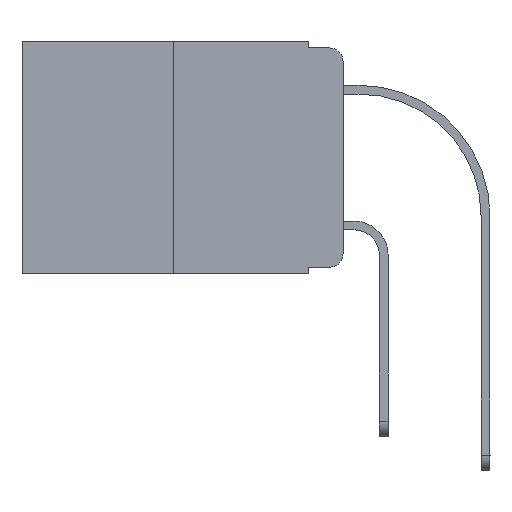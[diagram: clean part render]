
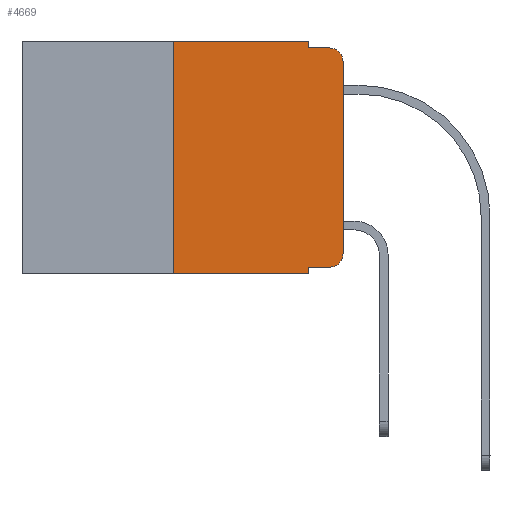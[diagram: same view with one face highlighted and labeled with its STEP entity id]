
A CAD part, left-side view. The second image highlights one B-rep face of the part: STEP entity #4669.
In plain terms, the highlighted planar face has unit normal (-1, 0, 0).
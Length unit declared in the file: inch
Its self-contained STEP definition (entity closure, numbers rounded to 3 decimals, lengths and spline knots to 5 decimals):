
#262 = DIRECTION ( 'NONE',  ( 0., 0., -1. ) ) ;
#368 = CIRCLE ( 'NONE', #6125, 0.02 ) ;
#521 = DIRECTION ( 'NONE',  ( 0., -1., 0. ) ) ;
#764 = CARTESIAN_POINT ( 'NONE',  ( 0., 0.25, 0. ) ) ;
#827 = EDGE_CURVE ( 'NONE', #19332, #5229, #12597, .T. ) ;
#1513 = VERTEX_POINT ( 'NONE', #13084 ) ;
#1625 = EDGE_CURVE ( 'NONE', #12214, #4567, #8659, .T. ) ;
#1886 = CIRCLE ( 'NONE', #13680, 0.02 ) ;
#1904 = VECTOR ( 'NONE', #11044, 39.37008 ) ;
#2000 = CARTESIAN_POINT ( 'NONE',  ( 0., 0.051, -0.333 ) ) ;
#2262 = EDGE_CURVE ( 'NONE', #12214, #17678, #7145, .T. ) ;
#3136 = DIRECTION ( 'NONE',  ( 0., -1., 0. ) ) ;
#3420 = ORIENTED_EDGE ( 'NONE', *, *, #6524, .F. ) ;
#3821 = CARTESIAN_POINT ( 'NONE',  ( 0., 0., -0.03 ) ) ;
#3942 = LINE ( 'NONE', #16697, #20056 ) ;
#4567 = VERTEX_POINT ( 'NONE', #17156 ) ;
#4573 = DIRECTION ( 'NONE',  ( 0., 0., 1. ) ) ;
#4669 = ADVANCED_FACE ( 'NONE', ( #4906 ), #11142, .F. ) ;
#4838 = VERTEX_POINT ( 'NONE', #14924 ) ;
#4906 = FACE_OUTER_BOUND ( 'NONE', #20108, .T. ) ;
#5229 = VERTEX_POINT ( 'NONE', #764 ) ;
#5810 = EDGE_CURVE ( 'NONE', #5229, #1513, #15790, .T. ) ;
#6083 = DIRECTION ( 'NONE',  ( 0., -1., 0. ) ) ;
#6125 = AXIS2_PLACEMENT_3D ( 'NONE', #7836, #12792, #10896 ) ;
#6155 = DIRECTION ( 'NONE',  ( 0., 0., -1. ) ) ;
#6524 = EDGE_CURVE ( 'NONE', #1513, #15358, #3942, .T. ) ;
#6560 = VECTOR ( 'NONE', #14799, 39.37008 ) ;
#7093 = DIRECTION ( 'NONE',  ( 0., 0., -1. ) ) ;
#7145 = LINE ( 'NONE', #9455, #1904 ) ;
#7532 = DIRECTION ( 'NONE',  ( 0., -1., 0. ) ) ;
#7761 = VERTEX_POINT ( 'NONE', #11628 ) ;
#7836 = CARTESIAN_POINT ( 'NONE',  ( 0., 0.02, -0.03 ) ) ;
#8020 = ORIENTED_EDGE ( 'NONE', *, *, #5810, .F. ) ;
#8023 = CARTESIAN_POINT ( 'NONE',  ( 0., 0.25, -0.343 ) ) ;
#8470 = CARTESIAN_POINT ( 'NONE',  ( 0., 0., 0. ) ) ;
#8659 = LINE ( 'NONE', #2000, #18472 ) ;
#9040 = EDGE_CURVE ( 'NONE', #4838, #12448, #11527, .T. ) ;
#9397 = ORIENTED_EDGE ( 'NONE', *, *, #20646, .F. ) ;
#9430 = ORIENTED_EDGE ( 'NONE', *, *, #827, .F. ) ;
#9455 = CARTESIAN_POINT ( 'NONE',  ( 0., 0.051, 0. ) ) ;
#10097 = ORIENTED_EDGE ( 'NONE', *, *, #9040, .T. ) ;
#10896 = DIRECTION ( 'NONE',  ( 0., 0., -1. ) ) ;
#11007 = ORIENTED_EDGE ( 'NONE', *, *, #11699, .T. ) ;
#11044 = DIRECTION ( 'NONE',  ( 0., 0., -1. ) ) ;
#11142 = PLANE ( 'NONE',  #19869 ) ;
#11153 = LINE ( 'NONE', #15801, #12660 ) ;
#11527 = LINE ( 'NONE', #8470, #6560 ) ;
#11628 = CARTESIAN_POINT ( 'NONE',  ( 0., 0.02, -0.01 ) ) ;
#11699 = EDGE_CURVE ( 'NONE', #19332, #17678, #11153, .T. ) ;
#12214 = VERTEX_POINT ( 'NONE', #13014 ) ;
#12390 = CARTESIAN_POINT ( 'NONE',  ( 0., 0.25, 0. ) ) ;
#12448 = VERTEX_POINT ( 'NONE', #3821 ) ;
#12595 = CARTESIAN_POINT ( 'NONE',  ( 0., 0.051, -0.01 ) ) ;
#12597 = LINE ( 'NONE', #12390, #19564 ) ;
#12660 = VECTOR ( 'NONE', #3136, 39.37008 ) ;
#12699 = CARTESIAN_POINT ( 'NONE',  ( 0., 0.051, -0.01 ) ) ;
#12792 = DIRECTION ( 'NONE',  ( -1., 0., 0. ) ) ;
#13014 = CARTESIAN_POINT ( 'NONE',  ( 0., 0.051, -0.333 ) ) ;
#13084 = CARTESIAN_POINT ( 'NONE',  ( 0., 0.051, 0. ) ) ;
#13507 = ORIENTED_EDGE ( 'NONE', *, *, #2262, .F. ) ;
#13570 = DIRECTION ( 'NONE',  ( -1., 0., 0. ) ) ;
#13680 = AXIS2_PLACEMENT_3D ( 'NONE', #15755, #13570, #6155 ) ;
#13827 = ORIENTED_EDGE ( 'NONE', *, *, #18657, .T. ) ;
#14082 = EDGE_CURVE ( 'NONE', #12448, #7761, #368, .T. ) ;
#14799 = DIRECTION ( 'NONE',  ( 0., 0., 1. ) ) ;
#14924 = CARTESIAN_POINT ( 'NONE',  ( 0., 0., -0.313 ) ) ;
#15358 = VERTEX_POINT ( 'NONE', #12699 ) ;
#15474 = CARTESIAN_POINT ( 'NONE',  ( 0., 0.473, 0. ) ) ;
#15719 = ORIENTED_EDGE ( 'NONE', *, *, #1625, .T. ) ;
#15755 = CARTESIAN_POINT ( 'NONE',  ( 0., 0.02, -0.313 ) ) ;
#15790 = LINE ( 'NONE', #15474, #18036 ) ;
#15801 = CARTESIAN_POINT ( 'NONE',  ( 0., 0.473, -0.343 ) ) ;
#16697 = CARTESIAN_POINT ( 'NONE',  ( 0., 0.051, 0. ) ) ;
#17156 = CARTESIAN_POINT ( 'NONE',  ( 0., 0.02, -0.333 ) ) ;
#17483 = ORIENTED_EDGE ( 'NONE', *, *, #14082, .T. ) ;
#17567 = DIRECTION ( 'NONE',  ( 1., 0., 0. ) ) ;
#17678 = VERTEX_POINT ( 'NONE', #19740 ) ;
#17782 = CARTESIAN_POINT ( 'NONE',  ( 0., 0.473, 0. ) ) ;
#17821 = VECTOR ( 'NONE', #7532, 39.37008 ) ;
#18036 = VECTOR ( 'NONE', #6083, 39.37008 ) ;
#18472 = VECTOR ( 'NONE', #521, 39.37008 ) ;
#18657 = EDGE_CURVE ( 'NONE', #4567, #4838, #1886, .T. ) ;
#19332 = VERTEX_POINT ( 'NONE', #8023 ) ;
#19564 = VECTOR ( 'NONE', #4573, 39.37008 ) ;
#19740 = CARTESIAN_POINT ( 'NONE',  ( 0., 0.051, -0.343 ) ) ;
#19869 = AXIS2_PLACEMENT_3D ( 'NONE', #17782, #17567, #262 ) ;
#20056 = VECTOR ( 'NONE', #7093, 39.37008 ) ;
#20108 = EDGE_LOOP ( 'NONE', ( #10097, #17483, #9397, #3420, #8020, #9430, #11007, #13507, #15719, #13827 ) ) ;
#20606 = LINE ( 'NONE', #12595, #17821 ) ;
#20646 = EDGE_CURVE ( 'NONE', #15358, #7761, #20606, .T. ) ;
